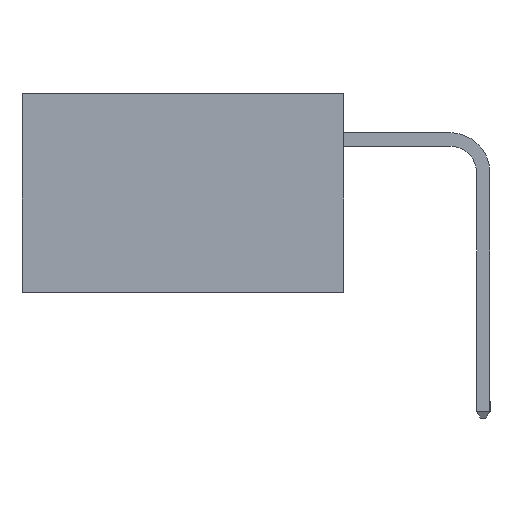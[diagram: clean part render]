
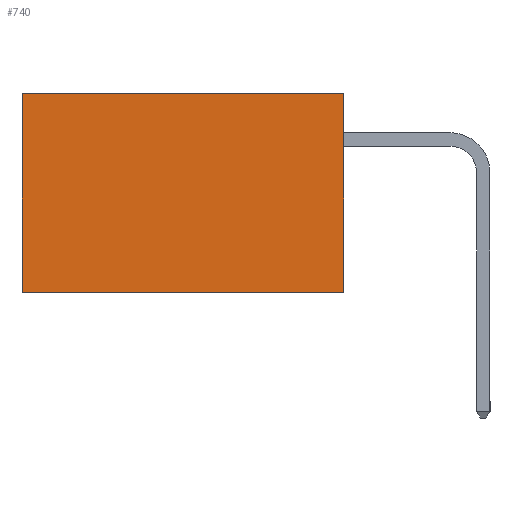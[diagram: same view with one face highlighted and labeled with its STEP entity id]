
A CAD part, left-side view. The second image highlights one B-rep face of the part: STEP entity #740.
In plain terms, the highlighted planar face has unit normal (-1, 0, 0).
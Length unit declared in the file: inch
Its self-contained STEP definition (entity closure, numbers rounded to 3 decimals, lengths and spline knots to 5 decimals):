
#740 = ADVANCED_FACE ( 'NONE', ( #10770 ), #2828, .F. ) ;
#929 = EDGE_CURVE ( 'NONE', #1976, #8663, #4938, .T. ) ;
#1407 = CARTESIAN_POINT ( 'NONE',  ( 0.2615, 0., -0.37 ) ) ;
#1484 = DIRECTION ( 'NONE',  ( 0., 0., -1. ) ) ;
#1976 = VERTEX_POINT ( 'NONE', #4386 ) ;
#2403 = LINE ( 'NONE', #8572, #9788 ) ;
#2611 = DIRECTION ( 'NONE',  ( 0., 0., -1. ) ) ;
#2828 = PLANE ( 'NONE',  #14257 ) ;
#3162 = VERTEX_POINT ( 'NONE', #11571 ) ;
#3184 = ORIENTED_EDGE ( 'NONE', *, *, #16819, .T. ) ;
#3653 = ORIENTED_EDGE ( 'NONE', *, *, #9729, .F. ) ;
#4386 = CARTESIAN_POINT ( 'NONE',  ( 0.2615, 0.6, 0. ) ) ;
#4938 = LINE ( 'NONE', #8483, #7989 ) ;
#5960 = ORIENTED_EDGE ( 'NONE', *, *, #16292, .F. ) ;
#6230 = LINE ( 'NONE', #9376, #15970 ) ;
#6285 = ORIENTED_EDGE ( 'NONE', *, *, #929, .T. ) ;
#6686 = DIRECTION ( 'NONE',  ( 0., 0., -1. ) ) ;
#7989 = VECTOR ( 'NONE', #2611, 39.37008 ) ;
#8483 = CARTESIAN_POINT ( 'NONE',  ( 0.2615, 0.6, -0.37 ) ) ;
#8524 = VERTEX_POINT ( 'NONE', #9224 ) ;
#8572 = CARTESIAN_POINT ( 'NONE',  ( 0.2615, 0., 0. ) ) ;
#8663 = VERTEX_POINT ( 'NONE', #13329 ) ;
#9224 = CARTESIAN_POINT ( 'NONE',  ( 0.2615, 0., -0.37 ) ) ;
#9376 = CARTESIAN_POINT ( 'NONE',  ( 0.2615, 0., -0.37 ) ) ;
#9729 = EDGE_CURVE ( 'NONE', #3162, #8524, #6230, .T. ) ;
#9788 = VECTOR ( 'NONE', #16137, 39.37008 ) ;
#10137 = CARTESIAN_POINT ( 'NONE',  ( 0.2615, 0., -0.37 ) ) ;
#10592 = LINE ( 'NONE', #10137, #14356 ) ;
#10770 = FACE_OUTER_BOUND ( 'NONE', #12257, .T. ) ;
#11402 = DIRECTION ( 'NONE',  ( 0., 1., 0. ) ) ;
#11571 = CARTESIAN_POINT ( 'NONE',  ( 0.2615, 0., 0. ) ) ;
#12257 = EDGE_LOOP ( 'NONE', ( #6285, #5960, #3653, #3184 ) ) ;
#13329 = CARTESIAN_POINT ( 'NONE',  ( 0.2615, 0.6, -0.37 ) ) ;
#14257 = AXIS2_PLACEMENT_3D ( 'NONE', #1407, #15634, #6686 ) ;
#14356 = VECTOR ( 'NONE', #11402, 39.37008 ) ;
#15634 = DIRECTION ( 'NONE',  ( 1., 0., 0. ) ) ;
#15970 = VECTOR ( 'NONE', #1484, 39.37008 ) ;
#16137 = DIRECTION ( 'NONE',  ( 0., 1., 0. ) ) ;
#16292 = EDGE_CURVE ( 'NONE', #8524, #8663, #10592, .T. ) ;
#16819 = EDGE_CURVE ( 'NONE', #3162, #1976, #2403, .T. ) ;
